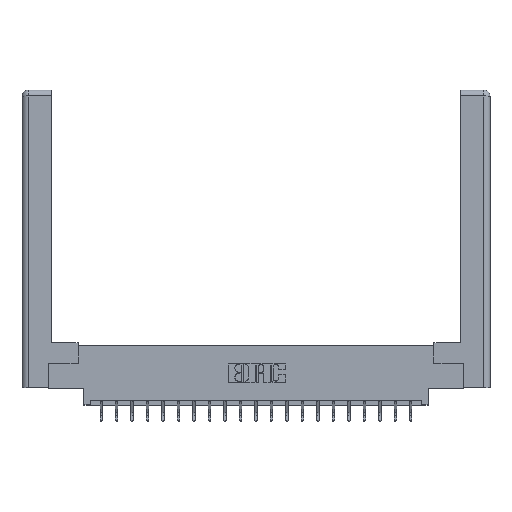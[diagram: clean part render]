
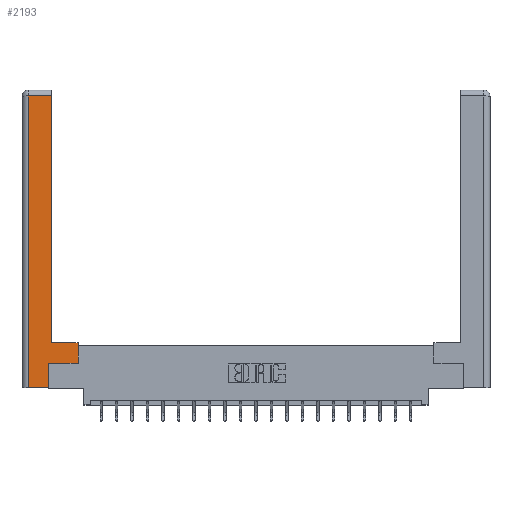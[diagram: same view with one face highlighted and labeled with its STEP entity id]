
A CAD part, top view. The second image highlights one B-rep face of the part: STEP entity #2193.
In plain terms, the highlighted planar face has unit normal (0, 0, 1).
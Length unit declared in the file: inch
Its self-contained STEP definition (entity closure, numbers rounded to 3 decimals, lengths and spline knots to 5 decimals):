
#68 = CARTESIAN_POINT ( 'NONE',  ( 0.565, 0.45, 0. ) ) ;
#306 = CARTESIAN_POINT ( 'NONE',  ( 0.295, 3., 0. ) ) ;
#486 = CARTESIAN_POINT ( 'NONE',  ( 0.265, 0.245, 0. ) ) ;
#1315 = VERTEX_POINT ( 'NONE', #21358 ) ;
#1456 = VERTEX_POINT ( 'NONE', #20821 ) ;
#1902 = CARTESIAN_POINT ( 'NONE',  ( 0.265, 0., 0. ) ) ;
#2193 = ADVANCED_FACE ( 'NONE', ( #2254 ), #3686, .F. ) ;
#2215 = DIRECTION ( 'NONE',  ( -1., 0., 0. ) ) ;
#2254 = FACE_OUTER_BOUND ( 'NONE', #16352, .T. ) ;
#2268 = EDGE_CURVE ( 'NONE', #1315, #17643, #4134, .T. ) ;
#3025 = LINE ( 'NONE', #306, #7036 ) ;
#3269 = CARTESIAN_POINT ( 'NONE',  ( 0.0615, 2.94, 0. ) ) ;
#3686 = PLANE ( 'NONE',  #18930 ) ;
#4134 = LINE ( 'NONE', #12705, #8648 ) ;
#4332 = CARTESIAN_POINT ( 'NONE',  ( 0.265, 0., 0. ) ) ;
#4555 = DIRECTION ( 'NONE',  ( 1., 0., 0. ) ) ;
#5036 = EDGE_CURVE ( 'NONE', #17795, #19095, #15615, .T. ) ;
#5265 = VECTOR ( 'NONE', #8617, 39.37008 ) ;
#5376 = VERTEX_POINT ( 'NONE', #12380 ) ;
#5574 = ORIENTED_EDGE ( 'NONE', *, *, #2268, .T. ) ;
#6226 = VERTEX_POINT ( 'NONE', #1902 ) ;
#6297 = LINE ( 'NONE', #7884, #7883 ) ;
#6878 = VECTOR ( 'NONE', #17088, 39.37008 ) ;
#7036 = VECTOR ( 'NONE', #10355, 39.37008 ) ;
#7198 = EDGE_CURVE ( 'NONE', #19095, #10647, #15619, .T. ) ;
#7317 = ORIENTED_EDGE ( 'NONE', *, *, #17728, .T. ) ;
#7883 = VECTOR ( 'NONE', #16092, 39.37008 ) ;
#7884 = CARTESIAN_POINT ( 'NONE',  ( 0.265, 0.245, 0. ) ) ;
#8449 = LINE ( 'NONE', #3269, #5265 ) ;
#8617 = DIRECTION ( 'NONE',  ( -1., 0., 0. ) ) ;
#8648 = VECTOR ( 'NONE', #17675, 39.37008 ) ;
#8769 = EDGE_CURVE ( 'NONE', #6226, #17795, #6297, .T. ) ;
#10096 = ORIENTED_EDGE ( 'NONE', *, *, #17580, .T. ) ;
#10170 = CARTESIAN_POINT ( 'NONE',  ( 0.565, 0.245, 0. ) ) ;
#10355 = DIRECTION ( 'NONE',  ( 0., 1., 0. ) ) ;
#10647 = VERTEX_POINT ( 'NONE', #11681 ) ;
#11681 = CARTESIAN_POINT ( 'NONE',  ( 0.565, 0.45, 0. ) ) ;
#11978 = ORIENTED_EDGE ( 'NONE', *, *, #7198, .T. ) ;
#12037 = DIRECTION ( 'NONE',  ( 0., 1., 0. ) ) ;
#12155 = VECTOR ( 'NONE', #4555, 39.37008 ) ;
#12380 = CARTESIAN_POINT ( 'NONE',  ( 0.295, 0.45, 0. ) ) ;
#12455 = VECTOR ( 'NONE', #12037, 39.37008 ) ;
#12600 = CARTESIAN_POINT ( 'NONE',  ( 0.295, 0.45, 0. ) ) ;
#12705 = CARTESIAN_POINT ( 'NONE',  ( 0.0615, 0., 0. ) ) ;
#13956 = EDGE_CURVE ( 'NONE', #5376, #1456, #3025, .T. ) ;
#14271 = DIRECTION ( 'NONE',  ( 0., 0., -1. ) ) ;
#15156 = ORIENTED_EDGE ( 'NONE', *, *, #8769, .T. ) ;
#15615 = LINE ( 'NONE', #10170, #6878 ) ;
#15619 = LINE ( 'NONE', #68, #12455 ) ;
#16092 = DIRECTION ( 'NONE',  ( 0., 1., 0. ) ) ;
#16352 = EDGE_LOOP ( 'NONE', ( #17429, #7317, #5574, #10096, #15156, #19445, #11978, #18270 ) ) ;
#17039 = LINE ( 'NONE', #12600, #21046 ) ;
#17088 = DIRECTION ( 'NONE',  ( 1., 0., 0. ) ) ;
#17429 = ORIENTED_EDGE ( 'NONE', *, *, #13956, .T. ) ;
#17528 = CARTESIAN_POINT ( 'NONE',  ( 0.565, 0.245, 0. ) ) ;
#17580 = EDGE_CURVE ( 'NONE', #17643, #6226, #18253, .T. ) ;
#17643 = VERTEX_POINT ( 'NONE', #18445 ) ;
#17675 = DIRECTION ( 'NONE',  ( 0., -1., 0. ) ) ;
#17728 = EDGE_CURVE ( 'NONE', #1456, #1315, #8449, .T. ) ;
#17795 = VERTEX_POINT ( 'NONE', #486 ) ;
#18253 = LINE ( 'NONE', #4332, #12155 ) ;
#18270 = ORIENTED_EDGE ( 'NONE', *, *, #20962, .T. ) ;
#18445 = CARTESIAN_POINT ( 'NONE',  ( 0.0615, 0., 0. ) ) ;
#18930 = AXIS2_PLACEMENT_3D ( 'NONE', #19630, #14271, #19557 ) ;
#19095 = VERTEX_POINT ( 'NONE', #17528 ) ;
#19445 = ORIENTED_EDGE ( 'NONE', *, *, #5036, .T. ) ;
#19557 = DIRECTION ( 'NONE',  ( -1., 0., 0. ) ) ;
#19630 = CARTESIAN_POINT ( 'NONE',  ( 0., 0., 0. ) ) ;
#20821 = CARTESIAN_POINT ( 'NONE',  ( 0.295, 2.94, 0. ) ) ;
#20962 = EDGE_CURVE ( 'NONE', #10647, #5376, #17039, .T. ) ;
#21046 = VECTOR ( 'NONE', #2215, 39.37008 ) ;
#21358 = CARTESIAN_POINT ( 'NONE',  ( 0.0615, 2.94, 0. ) ) ;
